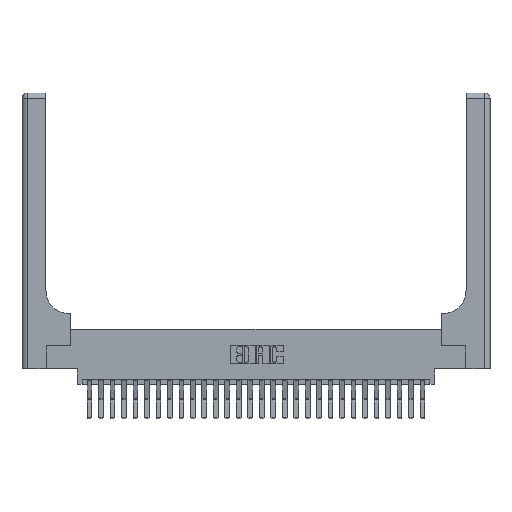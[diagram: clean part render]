
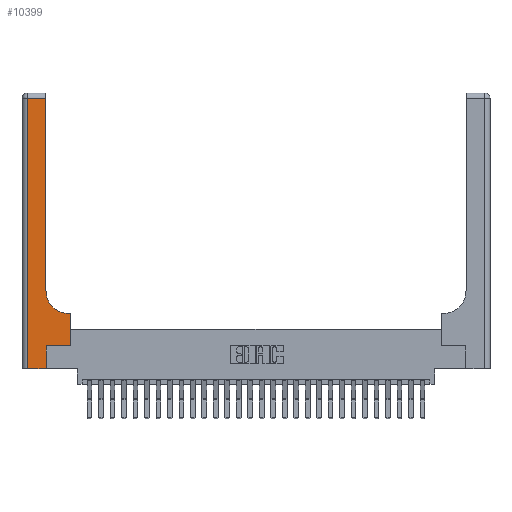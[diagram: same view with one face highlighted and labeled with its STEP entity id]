
A CAD part, top view. The second image highlights one B-rep face of the part: STEP entity #10399.
In plain terms, the highlighted planar face has unit normal (0, 0, 1).
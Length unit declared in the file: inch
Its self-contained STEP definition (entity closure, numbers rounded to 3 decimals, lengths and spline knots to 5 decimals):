
#2 = CARTESIAN_POINT ( 'NONE',  ( 0.26, 0.6, 0.37 ) ) ;
#877 = LINE ( 'NONE', #15168, #11865 ) ;
#1014 = CARTESIAN_POINT ( 'NONE',  ( 0.06, 3., 0.37 ) ) ;
#1203 = CARTESIAN_POINT ( 'NONE',  ( 0.26, 0.85, 0.37 ) ) ;
#1973 = VERTEX_POINT ( 'NONE', #1203 ) ;
#2166 = DIRECTION ( 'NONE',  ( 1., 0., 0. ) ) ;
#2346 = LINE ( 'NONE', #22465, #12693 ) ;
#2729 = EDGE_CURVE ( 'NONE', #15620, #22805, #21918, .T. ) ;
#2970 = CIRCLE ( 'NONE', #6468, 0.25 ) ;
#3225 = LINE ( 'NONE', #23727, #24440 ) ;
#3974 = DIRECTION ( 'NONE',  ( 0., 1., 0. ) ) ;
#4200 = LINE ( 'NONE', #2, #15176 ) ;
#4221 = CARTESIAN_POINT ( 'NONE',  ( 0., 3., 0.37 ) ) ;
#4275 = EDGE_CURVE ( 'NONE', #7181, #17644, #877, .T. ) ;
#4509 = CARTESIAN_POINT ( 'NONE',  ( 0.528, 0.6, 0.37 ) ) ;
#4803 = DIRECTION ( 'NONE',  ( 1., 0., 0. ) ) ;
#5328 = DIRECTION ( 'NONE',  ( 0., 1., 0. ) ) ;
#5350 = DIRECTION ( 'NONE',  ( -1., 0., 0. ) ) ;
#6081 = VECTOR ( 'NONE', #21587, 39.37008 ) ;
#6101 = DIRECTION ( 'NONE',  ( 0., 0., -1. ) ) ;
#6134 = DIRECTION ( 'NONE',  ( 0., 1., 0. ) ) ;
#6468 = AXIS2_PLACEMENT_3D ( 'NONE', #18399, #6101, #20436 ) ;
#6828 = CARTESIAN_POINT ( 'NONE',  ( 0.26, 2.94, 0.37 ) ) ;
#6888 = EDGE_CURVE ( 'NONE', #1973, #8789, #2346, .T. ) ;
#6938 = ORIENTED_EDGE ( 'NONE', *, *, #4275, .T. ) ;
#7181 = VERTEX_POINT ( 'NONE', #9021 ) ;
#8254 = VECTOR ( 'NONE', #2166, 39.37008 ) ;
#8587 = ORIENTED_EDGE ( 'NONE', *, *, #20800, .T. ) ;
#8789 = VERTEX_POINT ( 'NONE', #6828 ) ;
#8843 = ORIENTED_EDGE ( 'NONE', *, *, #11359, .T. ) ;
#9021 = CARTESIAN_POINT ( 'NONE',  ( 0.06, 0., 0.37 ) ) ;
#9038 = VERTEX_POINT ( 'NONE', #15752 ) ;
#9981 = ORIENTED_EDGE ( 'NONE', *, *, #2729, .T. ) ;
#10212 = CARTESIAN_POINT ( 'NONE',  ( 0.528, 0.25, 0.37 ) ) ;
#10311 = FACE_OUTER_BOUND ( 'NONE', #20745, .T. ) ;
#10399 = ADVANCED_FACE ( 'NONE', ( #10311 ), #10473, .F. ) ;
#10473 = PLANE ( 'NONE',  #24659 ) ;
#11091 = ORIENTED_EDGE ( 'NONE', *, *, #25956, .T. ) ;
#11359 = EDGE_CURVE ( 'NONE', #18372, #15620, #24573, .T. ) ;
#11566 = LINE ( 'NONE', #1014, #6081 ) ;
#11865 = VECTOR ( 'NONE', #4803, 39.37008 ) ;
#12470 = EDGE_CURVE ( 'NONE', #9038, #1973, #2970, .T. ) ;
#12526 = DIRECTION ( 'NONE',  ( -1., 0., 0. ) ) ;
#12545 = VERTEX_POINT ( 'NONE', #18647 ) ;
#12693 = VECTOR ( 'NONE', #3974, 39.37008 ) ;
#13524 = CARTESIAN_POINT ( 'NONE',  ( 0.265, 0., 0.37 ) ) ;
#14545 = CARTESIAN_POINT ( 'NONE',  ( 0.265, 0.25, 0.37 ) ) ;
#14806 = LINE ( 'NONE', #13524, #19565 ) ;
#14884 = CARTESIAN_POINT ( 'NONE',  ( 0.528, 0.25, 0.37 ) ) ;
#15168 = CARTESIAN_POINT ( 'NONE',  ( 0., 0., 0.37 ) ) ;
#15176 = VECTOR ( 'NONE', #20509, 39.37008 ) ;
#15358 = ORIENTED_EDGE ( 'NONE', *, *, #12470, .T. ) ;
#15538 = ORIENTED_EDGE ( 'NONE', *, *, #6888, .T. ) ;
#15620 = VERTEX_POINT ( 'NONE', #14884 ) ;
#15752 = CARTESIAN_POINT ( 'NONE',  ( 0.51, 0.6, 0.37 ) ) ;
#15856 = EDGE_CURVE ( 'NONE', #17644, #18372, #14806, .T. ) ;
#16515 = VECTOR ( 'NONE', #6134, 39.37008 ) ;
#17231 = CARTESIAN_POINT ( 'NONE',  ( 0.265, 0., 0.37 ) ) ;
#17391 = ORIENTED_EDGE ( 'NONE', *, *, #15856, .T. ) ;
#17644 = VERTEX_POINT ( 'NONE', #17231 ) ;
#18372 = VERTEX_POINT ( 'NONE', #26003 ) ;
#18399 = CARTESIAN_POINT ( 'NONE',  ( 0.51, 0.85, 0.37 ) ) ;
#18647 = CARTESIAN_POINT ( 'NONE',  ( 0.06, 2.94, 0.37 ) ) ;
#19565 = VECTOR ( 'NONE', #5328, 39.37008 ) ;
#20436 = DIRECTION ( 'NONE',  ( 1., 0., 0. ) ) ;
#20509 = DIRECTION ( 'NONE',  ( -1., 0., 0. ) ) ;
#20745 = EDGE_LOOP ( 'NONE', ( #15538, #8587, #25591, #6938, #17391, #8843, #9981, #11091, #15358 ) ) ;
#20800 = EDGE_CURVE ( 'NONE', #8789, #12545, #3225, .T. ) ;
#21587 = DIRECTION ( 'NONE',  ( 0., -1., 0. ) ) ;
#21918 = LINE ( 'NONE', #10212, #16515 ) ;
#22373 = EDGE_CURVE ( 'NONE', #12545, #7181, #11566, .T. ) ;
#22465 = CARTESIAN_POINT ( 'NONE',  ( 0.26, 3., 0.37 ) ) ;
#22805 = VERTEX_POINT ( 'NONE', #4509 ) ;
#23727 = CARTESIAN_POINT ( 'NONE',  ( 0., 2.94, 0.37 ) ) ;
#24440 = VECTOR ( 'NONE', #5350, 39.37008 ) ;
#24573 = LINE ( 'NONE', #14545, #8254 ) ;
#24659 = AXIS2_PLACEMENT_3D ( 'NONE', #4221, #24772, #12526 ) ;
#24772 = DIRECTION ( 'NONE',  ( 0., 0., -1. ) ) ;
#25591 = ORIENTED_EDGE ( 'NONE', *, *, #22373, .T. ) ;
#25956 = EDGE_CURVE ( 'NONE', #22805, #9038, #4200, .T. ) ;
#26003 = CARTESIAN_POINT ( 'NONE',  ( 0.265, 0.25, 0.37 ) ) ;
